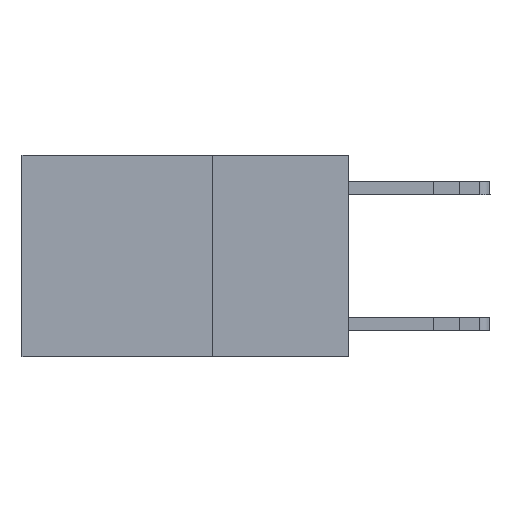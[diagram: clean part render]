
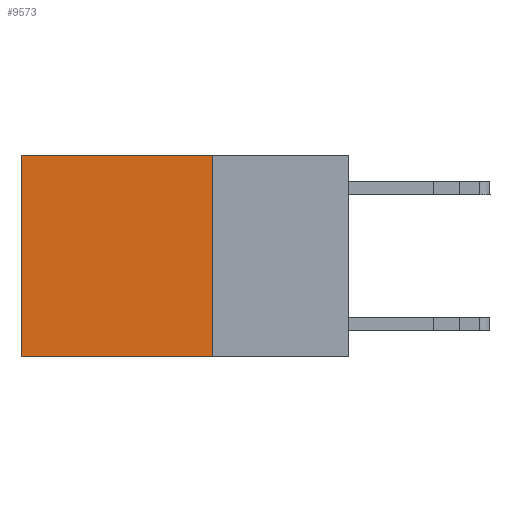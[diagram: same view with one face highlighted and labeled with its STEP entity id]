
A CAD part, left-side view. The second image highlights one B-rep face of the part: STEP entity #9573.
In plain terms, the highlighted planar face has unit normal (-1, 0, 0).
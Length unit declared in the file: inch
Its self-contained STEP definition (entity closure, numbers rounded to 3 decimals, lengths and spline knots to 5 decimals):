
#229 = LINE ( 'NONE', #6458, #13310 ) ;
#280 = VERTEX_POINT ( 'NONE', #13284 ) ;
#631 = ORIENTED_EDGE ( 'NONE', *, *, #8307, .T. ) ;
#919 = LINE ( 'NONE', #7837, #9047 ) ;
#1198 = VERTEX_POINT ( 'NONE', #8511 ) ;
#1415 = DIRECTION ( 'NONE',  ( 0., 0., -1. ) ) ;
#1950 = EDGE_CURVE ( 'NONE', #280, #7673, #229, .T. ) ;
#2775 = DIRECTION ( 'NONE',  ( 1., 0., 0. ) ) ;
#2877 = CARTESIAN_POINT ( 'NONE',  ( 0.2625, 0.25, -0.37 ) ) ;
#3272 = ORIENTED_EDGE ( 'NONE', *, *, #13118, .F. ) ;
#3856 = PLANE ( 'NONE',  #12351 ) ;
#4007 = DIRECTION ( 'NONE',  ( 0., 1., 0. ) ) ;
#4100 = VECTOR ( 'NONE', #6280, 39.37008 ) ;
#5103 = ORIENTED_EDGE ( 'NONE', *, *, #11572, .F. ) ;
#5367 = VERTEX_POINT ( 'NONE', #5575 ) ;
#5575 = CARTESIAN_POINT ( 'NONE',  ( 0.2625, 0.25, -0.37 ) ) ;
#6280 = DIRECTION ( 'NONE',  ( 0., 1., 0. ) ) ;
#6391 = DIRECTION ( 'NONE',  ( 0., 0., -1. ) ) ;
#6458 = CARTESIAN_POINT ( 'NONE',  ( 0.2625, 0.6, 0. ) ) ;
#7014 = FACE_OUTER_BOUND ( 'NONE', #10888, .T. ) ;
#7673 = VERTEX_POINT ( 'NONE', #8029 ) ;
#7837 = CARTESIAN_POINT ( 'NONE',  ( 0.2625, 0.25, 0. ) ) ;
#8029 = CARTESIAN_POINT ( 'NONE',  ( 0.2625, 0.6, -0.37 ) ) ;
#8136 = LINE ( 'NONE', #13033, #10793 ) ;
#8307 = EDGE_CURVE ( 'NONE', #1198, #280, #8136, .T. ) ;
#8511 = CARTESIAN_POINT ( 'NONE',  ( 0.2625, 0.25, 0. ) ) ;
#8747 = ORIENTED_EDGE ( 'NONE', *, *, #1950, .T. ) ;
#9047 = VECTOR ( 'NONE', #1415, 39.37008 ) ;
#9054 = CARTESIAN_POINT ( 'NONE',  ( 0.2625, 0.25, 0. ) ) ;
#9573 = ADVANCED_FACE ( 'NONE', ( #7014 ), #3856, .F. ) ;
#10028 = DIRECTION ( 'NONE',  ( 0., 0., -1. ) ) ;
#10793 = VECTOR ( 'NONE', #4007, 39.37008 ) ;
#10888 = EDGE_LOOP ( 'NONE', ( #8747, #5103, #3272, #631 ) ) ;
#11572 = EDGE_CURVE ( 'NONE', #5367, #7673, #12160, .T. ) ;
#12160 = LINE ( 'NONE', #2877, #4100 ) ;
#12351 = AXIS2_PLACEMENT_3D ( 'NONE', #9054, #2775, #10028 ) ;
#13033 = CARTESIAN_POINT ( 'NONE',  ( 0.2625, 0.25, 0. ) ) ;
#13118 = EDGE_CURVE ( 'NONE', #1198, #5367, #919, .T. ) ;
#13284 = CARTESIAN_POINT ( 'NONE',  ( 0.2625, 0.6, 0. ) ) ;
#13310 = VECTOR ( 'NONE', #6391, 39.37008 ) ;
